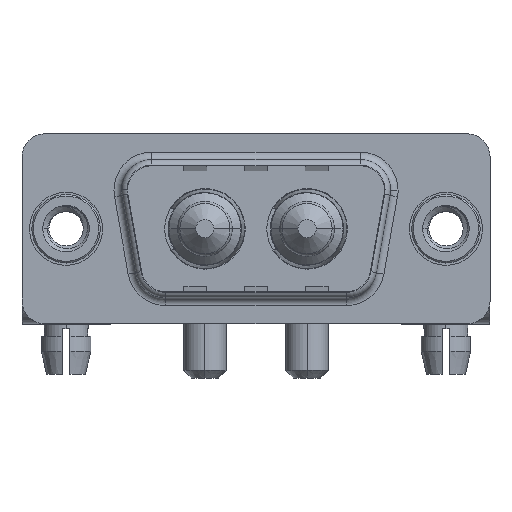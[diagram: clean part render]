
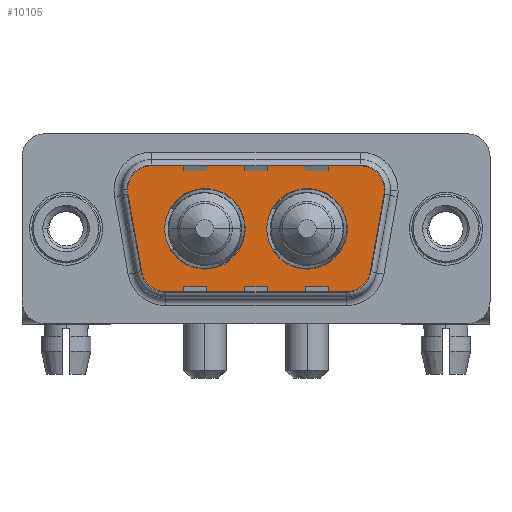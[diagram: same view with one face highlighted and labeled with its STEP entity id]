
A CAD part, top view. The second image highlights one B-rep face of the part: STEP entity #10105.
In plain terms, the highlighted planar face has unit normal (0, 0, 1).
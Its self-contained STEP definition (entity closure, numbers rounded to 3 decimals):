
#82 = ORIENTED_EDGE ( 'NONE', *, *, #2116, .T. ) ;
#341 = EDGE_CURVE ( 'NONE', #11591, #13862, #13534, .T. ) ;
#569 = AXIS2_PLACEMENT_3D ( 'NONE', #10420, #6679, #885 ) ;
#638 = EDGE_CURVE ( 'NONE', #8777, #8926, #2350, .T. ) ;
#790 = VERTEX_POINT ( 'NONE', #12256 ) ;
#847 = CIRCLE ( 'NONE', #569, 2. ) ;
#885 = DIRECTION ( 'NONE',  ( -1., 0., 0. ) ) ;
#1002 = ORIENTED_EDGE ( 'NONE', *, *, #8605, .T. ) ;
#1041 = ORIENTED_EDGE ( 'NONE', *, *, #1637, .F. ) ;
#1257 = AXIS2_PLACEMENT_3D ( 'NONE', #9974, #4250, #9904 ) ;
#1599 = CARTESIAN_POINT ( 'NONE',  ( 15.86, 0., 0. ) ) ;
#1607 = DIRECTION ( 'NONE',  ( -1., 0., 0. ) ) ;
#1637 = EDGE_CURVE ( 'NONE', #7348, #7038, #10886, .T. ) ;
#1747 = CARTESIAN_POINT ( 'NONE',  ( 15.86, 0., 0. ) ) ;
#2011 = DIRECTION ( 'NONE',  ( 1., 0., 0. ) ) ;
#2116 = EDGE_CURVE ( 'NONE', #7294, #7613, #10240, .T. ) ;
#2254 = CARTESIAN_POINT ( 'NONE',  ( 18.541, -4.9, 0. ) ) ;
#2350 = LINE ( 'NONE', #7011, #11597 ) ;
#2367 = CIRCLE ( 'NONE', #7003, 2.65 ) ;
#2543 = CIRCLE ( 'NONE', #8632, 2.65 ) ;
#2660 = CARTESIAN_POINT ( 'NONE',  ( 6.459, -2.9, 0. ) ) ;
#2821 = DIRECTION ( 'NONE',  ( 0., 0., 1. ) ) ;
#3309 = LINE ( 'NONE', #14897, #4989 ) ;
#3492 = ORIENTED_EDGE ( 'NONE', *, *, #9368, .T. ) ;
#3777 = AXIS2_PLACEMENT_3D ( 'NONE', #12401, #10100, #14753 ) ;
#3802 = CARTESIAN_POINT ( 'NONE',  ( 5.436, 2.9, 0. ) ) ;
#4229 = ORIENTED_EDGE ( 'NONE', *, *, #341, .F. ) ;
#4250 = DIRECTION ( 'NONE',  ( 0., 0., 1. ) ) ;
#4404 = CARTESIAN_POINT ( 'NONE',  ( 6.459, -4.9, 0. ) ) ;
#4858 = CIRCLE ( 'NONE', #5092, 2. ) ;
#4876 = DIRECTION ( 'NONE',  ( 1., 0., 0. ) ) ;
#4900 = CARTESIAN_POINT ( 'NONE',  ( 5.436, 4.9, 0. ) ) ;
#4910 = ORIENTED_EDGE ( 'NONE', *, *, #638, .T. ) ;
#4989 = VECTOR ( 'NONE', #10545, 1000. ) ;
#5076 = ORIENTED_EDGE ( 'NONE', *, *, #13022, .F. ) ;
#5092 = AXIS2_PLACEMENT_3D ( 'NONE', #3802, #8459, #13106 ) ;
#5230 = AXIS2_PLACEMENT_3D ( 'NONE', #12444, #5509, #9017 ) ;
#5400 = CARTESIAN_POINT ( 'NONE',  ( 21.534, 2.553, 0. ) ) ;
#5405 = DIRECTION ( 'NONE',  ( 1., 0., 0. ) ) ;
#5509 = DIRECTION ( 'NONE',  ( 0., 0., 1. ) ) ;
#5681 = DIRECTION ( 'NONE',  ( 0., 0., 1. ) ) ;
#5803 = DIRECTION ( 'NONE',  ( 0., 0., 1. ) ) ;
#6110 = ORIENTED_EDGE ( 'NONE', *, *, #9459, .T. ) ;
#6442 = CIRCLE ( 'NONE', #5230, 2. ) ;
#6524 = CARTESIAN_POINT ( 'NONE',  ( 9.14, 0., 0. ) ) ;
#6679 = DIRECTION ( 'NONE',  ( 0., 0., 1. ) ) ;
#6752 = AXIS2_PLACEMENT_3D ( 'NONE', #11469, #5681, #9265 ) ;
#7003 = AXIS2_PLACEMENT_3D ( 'NONE', #6524, #8667, #2011 ) ;
#7011 = CARTESIAN_POINT ( 'NONE',  ( 6.459, -4.9, 0. ) ) ;
#7038 = VERTEX_POINT ( 'NONE', #11894 ) ;
#7104 = LINE ( 'NONE', #4900, #14983 ) ;
#7172 = EDGE_CURVE ( 'NONE', #7038, #7348, #2367, .T. ) ;
#7294 = VERTEX_POINT ( 'NONE', #13529 ) ;
#7348 = VERTEX_POINT ( 'NONE', #15063 ) ;
#7613 = VERTEX_POINT ( 'NONE', #14372 ) ;
#8069 = CARTESIAN_POINT ( 'NONE',  ( 19.564, 4.9, 0. ) ) ;
#8116 = ORIENTED_EDGE ( 'NONE', *, *, #13845, .T. ) ;
#8256 = AXIS2_PLACEMENT_3D ( 'NONE', #2660, #5803, #11666 ) ;
#8434 = AXIS2_PLACEMENT_3D ( 'NONE', #1747, #2821, #12136 ) ;
#8459 = DIRECTION ( 'NONE',  ( 0., 0., 1. ) ) ;
#8604 = EDGE_CURVE ( 'NONE', #14509, #7294, #4858, .T. ) ;
#8605 = EDGE_CURVE ( 'NONE', #7613, #8777, #11906, .T. ) ;
#8613 = FACE_BOUND ( 'NONE', #9820, .T. ) ;
#8632 = AXIS2_PLACEMENT_3D ( 'NONE', #1599, #11119, #5405 ) ;
#8667 = DIRECTION ( 'NONE',  ( 0., 0., 1. ) ) ;
#8777 = VERTEX_POINT ( 'NONE', #4404 ) ;
#8926 = VERTEX_POINT ( 'NONE', #2254 ) ;
#9017 = DIRECTION ( 'NONE',  ( -1., 0., 0. ) ) ;
#9194 = ORIENTED_EDGE ( 'NONE', *, *, #14623, .T. ) ;
#9265 = DIRECTION ( 'NONE',  ( 1., 0., 0. ) ) ;
#9368 = EDGE_CURVE ( 'NONE', #8926, #14288, #10349, .T. ) ;
#9459 = EDGE_CURVE ( 'NONE', #10290, #14509, #7104, .T. ) ;
#9820 = EDGE_LOOP ( 'NONE', ( #5076, #4229 ) ) ;
#9904 = DIRECTION ( 'NONE',  ( 1., 0., 0. ) ) ;
#9974 = CARTESIAN_POINT ( 'NONE',  ( 18.541, -2.9, 0. ) ) ;
#10100 = DIRECTION ( 'NONE',  ( 0., 0., 1. ) ) ;
#10105 = ADVANCED_FACE ( 'NONE', ( #8613, #14484, #13262 ), #12132, .T. ) ;
#10183 = VERTEX_POINT ( 'NONE', #5400 ) ;
#10240 = LINE ( 'NONE', #14658, #10658 ) ;
#10266 = CARTESIAN_POINT ( 'NONE',  ( 18.51, 0., 0. ) ) ;
#10290 = VERTEX_POINT ( 'NONE', #8069 ) ;
#10349 = CIRCLE ( 'NONE', #3777, 2. ) ;
#10420 = CARTESIAN_POINT ( 'NONE',  ( 19.564, 2.9, 0. ) ) ;
#10545 = DIRECTION ( 'NONE',  ( 0.174, 0.985, 0. ) ) ;
#10658 = VECTOR ( 'NONE', #14888, 1000. ) ;
#10795 = ORIENTED_EDGE ( 'NONE', *, *, #13324, .T. ) ;
#10886 = CIRCLE ( 'NONE', #6752, 2.65 ) ;
#10973 = ORIENTED_EDGE ( 'NONE', *, *, #8604, .T. ) ;
#11119 = DIRECTION ( 'NONE',  ( 0., 0., 1. ) ) ;
#11469 = CARTESIAN_POINT ( 'NONE',  ( 9.14, 0., 0. ) ) ;
#11591 = VERTEX_POINT ( 'NONE', #13638 ) ;
#11597 = VECTOR ( 'NONE', #4876, 1000. ) ;
#11666 = DIRECTION ( 'NONE',  ( -1., 0., 0. ) ) ;
#11894 = CARTESIAN_POINT ( 'NONE',  ( 11.79, 0., 0. ) ) ;
#11906 = CIRCLE ( 'NONE', #8256, 2. ) ;
#12132 = PLANE ( 'NONE',  #1257 ) ;
#12136 = DIRECTION ( 'NONE',  ( 1., 0., 0. ) ) ;
#12256 = CARTESIAN_POINT ( 'NONE',  ( 21.564, 2.9, 0. ) ) ;
#12401 = CARTESIAN_POINT ( 'NONE',  ( 18.541, -2.9, 0. ) ) ;
#12444 = CARTESIAN_POINT ( 'NONE',  ( 19.564, 2.9, 0. ) ) ;
#13022 = EDGE_CURVE ( 'NONE', #13862, #11591, #2543, .T. ) ;
#13106 = DIRECTION ( 'NONE',  ( 1., 0., 0. ) ) ;
#13262 = FACE_OUTER_BOUND ( 'NONE', #14256, .T. ) ;
#13293 = CARTESIAN_POINT ( 'NONE',  ( 5.436, 4.9, 0. ) ) ;
#13324 = EDGE_CURVE ( 'NONE', #14288, #10183, #3309, .T. ) ;
#13529 = CARTESIAN_POINT ( 'NONE',  ( 3.466, 2.553, 0. ) ) ;
#13534 = CIRCLE ( 'NONE', #8434, 2.65 ) ;
#13638 = CARTESIAN_POINT ( 'NONE',  ( 13.21, 0., 0. ) ) ;
#13678 = CARTESIAN_POINT ( 'NONE',  ( 20.511, -3.247, 0. ) ) ;
#13760 = EDGE_LOOP ( 'NONE', ( #14640, #1041 ) ) ;
#13845 = EDGE_CURVE ( 'NONE', #790, #10290, #847, .T. ) ;
#13862 = VERTEX_POINT ( 'NONE', #10266 ) ;
#14256 = EDGE_LOOP ( 'NONE', ( #3492, #10795, #9194, #8116, #6110, #10973, #82, #1002, #4910 ) ) ;
#14288 = VERTEX_POINT ( 'NONE', #13678 ) ;
#14372 = CARTESIAN_POINT ( 'NONE',  ( 4.489, -3.247, 0. ) ) ;
#14484 = FACE_BOUND ( 'NONE', #13760, .T. ) ;
#14509 = VERTEX_POINT ( 'NONE', #13293 ) ;
#14623 = EDGE_CURVE ( 'NONE', #10183, #790, #6442, .T. ) ;
#14640 = ORIENTED_EDGE ( 'NONE', *, *, #7172, .F. ) ;
#14658 = CARTESIAN_POINT ( 'NONE',  ( 3.466, 2.553, 0. ) ) ;
#14753 = DIRECTION ( 'NONE',  ( 1., 0., 0. ) ) ;
#14888 = DIRECTION ( 'NONE',  ( 0.174, -0.985, 0. ) ) ;
#14897 = CARTESIAN_POINT ( 'NONE',  ( 21.534, 2.553, 0. ) ) ;
#14983 = VECTOR ( 'NONE', #1607, 1000. ) ;
#15063 = CARTESIAN_POINT ( 'NONE',  ( 6.49, 0., 0. ) ) ;
